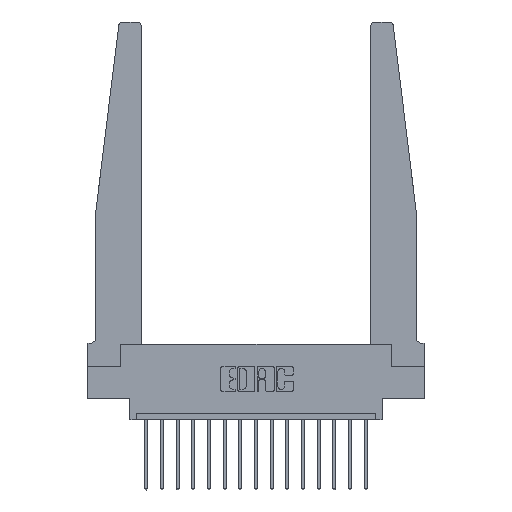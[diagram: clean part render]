
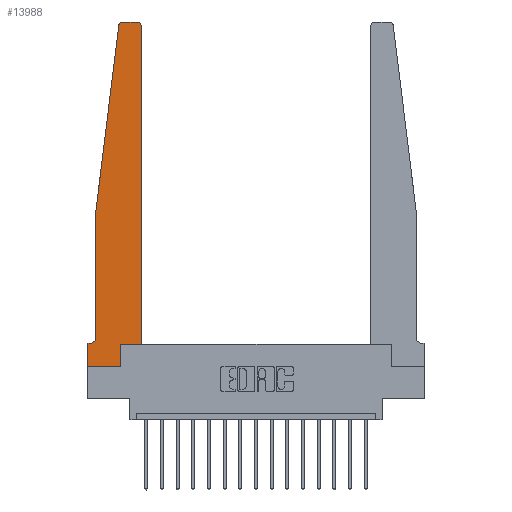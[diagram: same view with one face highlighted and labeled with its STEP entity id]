
A CAD part, top view. The second image highlights one B-rep face of the part: STEP entity #13988.
In plain terms, the highlighted planar face has unit normal (0, 0, 1).
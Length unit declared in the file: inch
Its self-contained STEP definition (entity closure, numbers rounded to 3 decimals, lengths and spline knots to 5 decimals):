
#480 = CARTESIAN_POINT ( 'NONE',  ( 0.065, 1.25, 0.37 ) ) ;
#621 = CARTESIAN_POINT ( 'NONE',  ( 0., 0.1875, 0.37 ) ) ;
#783 = CARTESIAN_POINT ( 'NONE',  ( 0.395, 2.75, 0.37 ) ) ;
#1248 = DIRECTION ( 'NONE',  ( 1., 0., 0. ) ) ;
#1488 = ORIENTED_EDGE ( 'NONE', *, *, #14935, .T. ) ;
#1908 = VERTEX_POINT ( 'NONE', #783 ) ;
#2038 = DIRECTION ( 'NONE',  ( -1., 0., 0. ) ) ;
#2104 = VERTEX_POINT ( 'NONE', #3308 ) ;
#2433 = ORIENTED_EDGE ( 'NONE', *, *, #8344, .T. ) ;
#2502 = LINE ( 'NONE', #14557, #13709 ) ;
#2522 = CIRCLE ( 'NONE', #10363, 0.05 ) ;
#2773 = VECTOR ( 'NONE', #1248, 39.37008 ) ;
#3038 = VERTEX_POINT ( 'NONE', #7591 ) ;
#3308 = CARTESIAN_POINT ( 'NONE',  ( 0., 0.1875, 0.37 ) ) ;
#3406 = CARTESIAN_POINT ( 'NONE',  ( 0.2605, 0.18, 0.37 ) ) ;
#3491 = VERTEX_POINT ( 'NONE', #6097 ) ;
#3689 = ORIENTED_EDGE ( 'NONE', *, *, #9313, .T. ) ;
#3926 = CARTESIAN_POINT ( 'NONE',  ( 0.065, 1.25, 0.37 ) ) ;
#4553 = VECTOR ( 'NONE', #16509, 39.37008 ) ;
#4703 = DIRECTION ( 'NONE',  ( 0., 1., 0. ) ) ;
#4928 = EDGE_CURVE ( 'NONE', #1908, #5959, #12519, .T. ) ;
#5096 = EDGE_CURVE ( 'NONE', #12871, #5785, #17444, .T. ) ;
#5451 = EDGE_CURVE ( 'NONE', #3491, #14314, #6489, .T. ) ;
#5543 = DIRECTION ( 'NONE',  ( 0., -1., 0. ) ) ;
#5785 = VERTEX_POINT ( 'NONE', #13978 ) ;
#5904 = ORIENTED_EDGE ( 'NONE', *, *, #12366, .T. ) ;
#5959 = VERTEX_POINT ( 'NONE', #14823 ) ;
#6097 = CARTESIAN_POINT ( 'NONE',  ( 0., 0., 0.37 ) ) ;
#6121 = DIRECTION ( 'NONE',  ( 0., 0., 1. ) ) ;
#6227 = DIRECTION ( 'NONE',  ( 0., 1., 0. ) ) ;
#6236 = CARTESIAN_POINT ( 'NONE',  ( 0.425, 2.72, 0.37 ) ) ;
#6269 = CARTESIAN_POINT ( 'NONE',  ( 0.015, 0.2375, 0.37 ) ) ;
#6274 = CARTESIAN_POINT ( 'NONE',  ( 0., 0., 0.37 ) ) ;
#6448 = DIRECTION ( 'NONE',  ( 1., 0., 0. ) ) ;
#6489 = LINE ( 'NONE', #6274, #15973 ) ;
#6546 = CARTESIAN_POINT ( 'NONE',  ( 0.24675, 2.72367, 0.37 ) ) ;
#6833 = CARTESIAN_POINT ( 'NONE',  ( 0.25, 2.75, 0.37 ) ) ;
#6857 = EDGE_CURVE ( 'NONE', #11253, #3038, #9467, .T. ) ;
#6870 = AXIS2_PLACEMENT_3D ( 'NONE', #11868, #9277, #6448 ) ;
#6974 = VERTEX_POINT ( 'NONE', #12579 ) ;
#6988 = AXIS2_PLACEMENT_3D ( 'NONE', #621, #6121, #8669 ) ;
#7047 = LINE ( 'NONE', #9644, #16525 ) ;
#7120 = DIRECTION ( 'NONE',  ( 1., 0., 0. ) ) ;
#7545 = CARTESIAN_POINT ( 'NONE',  ( 0.2605, 0.18, 0.37 ) ) ;
#7557 = EDGE_CURVE ( 'NONE', #2104, #3491, #7047, .T. ) ;
#7591 = CARTESIAN_POINT ( 'NONE',  ( 0.425, 0.18, 0.37 ) ) ;
#7655 = DIRECTION ( 'NONE',  ( 0., 0., -1. ) ) ;
#8344 = EDGE_CURVE ( 'NONE', #6974, #2104, #2502, .T. ) ;
#8518 = VECTOR ( 'NONE', #4703, 39.37008 ) ;
#8548 = ORIENTED_EDGE ( 'NONE', *, *, #16990, .T. ) ;
#8644 = LINE ( 'NONE', #7545, #16201 ) ;
#8669 = DIRECTION ( 'NONE',  ( 1., 0., 0. ) ) ;
#9277 = DIRECTION ( 'NONE',  ( 0., 0., 1. ) ) ;
#9313 = EDGE_CURVE ( 'NONE', #3038, #16264, #12194, .T. ) ;
#9467 = LINE ( 'NONE', #17684, #2773 ) ;
#9644 = CARTESIAN_POINT ( 'NONE',  ( 0., 0., 0.37 ) ) ;
#9719 = ORIENTED_EDGE ( 'NONE', *, *, #5451, .T. ) ;
#9935 = CARTESIAN_POINT ( 'NONE',  ( 0.2605, 0., 0.37 ) ) ;
#9998 = DIRECTION ( 'NONE',  ( 0., -1., 0. ) ) ;
#10363 = AXIS2_PLACEMENT_3D ( 'NONE', #6269, #7655, #17209 ) ;
#10529 = FACE_OUTER_BOUND ( 'NONE', #15155, .T. ) ;
#10700 = CIRCLE ( 'NONE', #16683, 0.03 ) ;
#10839 = LINE ( 'NONE', #17429, #15358 ) ;
#11007 = EDGE_CURVE ( 'NONE', #14314, #11253, #8644, .T. ) ;
#11041 = ORIENTED_EDGE ( 'NONE', *, *, #11007, .T. ) ;
#11253 = VERTEX_POINT ( 'NONE', #3406 ) ;
#11341 = DIRECTION ( 'NONE',  ( 0., 0., 1. ) ) ;
#11452 = ORIENTED_EDGE ( 'NONE', *, *, #5096, .T. ) ;
#11868 = CARTESIAN_POINT ( 'NONE',  ( 0.27653, 2.72, 0.37 ) ) ;
#12055 = CIRCLE ( 'NONE', #6870, 0.03 ) ;
#12194 = LINE ( 'NONE', #14048, #8518 ) ;
#12366 = EDGE_CURVE ( 'NONE', #5959, #14798, #12055, .T. ) ;
#12519 = LINE ( 'NONE', #6833, #4553 ) ;
#12579 = CARTESIAN_POINT ( 'NONE',  ( 0.015, 0.1875, 0.37 ) ) ;
#12871 = VERTEX_POINT ( 'NONE', #3926 ) ;
#13558 = EDGE_CURVE ( 'NONE', #5785, #6974, #2522, .T. ) ;
#13709 = VECTOR ( 'NONE', #2038, 39.37008 ) ;
#13826 = VECTOR ( 'NONE', #9998, 39.37008 ) ;
#13978 = CARTESIAN_POINT ( 'NONE',  ( 0.065, 0.2375, 0.37 ) ) ;
#13988 = ADVANCED_FACE ( 'NONE', ( #10529 ), #15545, .T. ) ;
#14048 = CARTESIAN_POINT ( 'NONE',  ( 0.425, 0.18, 0.37 ) ) ;
#14314 = VERTEX_POINT ( 'NONE', #9935 ) ;
#14557 = CARTESIAN_POINT ( 'NONE',  ( 0.065, 0.1875, 0.37 ) ) ;
#14798 = VERTEX_POINT ( 'NONE', #6546 ) ;
#14823 = CARTESIAN_POINT ( 'NONE',  ( 0.27653, 2.75, 0.37 ) ) ;
#14935 = EDGE_CURVE ( 'NONE', #16264, #1908, #10700, .T. ) ;
#15155 = EDGE_LOOP ( 'NONE', ( #15226, #5904, #8548, #11452, #17633, #2433, #17727, #9719, #11041, #15281, #3689, #1488 ) ) ;
#15226 = ORIENTED_EDGE ( 'NONE', *, *, #4928, .T. ) ;
#15281 = ORIENTED_EDGE ( 'NONE', *, *, #6857, .T. ) ;
#15358 = VECTOR ( 'NONE', #16026, 39.37008 ) ;
#15545 = PLANE ( 'NONE',  #6988 ) ;
#15973 = VECTOR ( 'NONE', #15980, 39.37008 ) ;
#15980 = DIRECTION ( 'NONE',  ( 1., 0., 0. ) ) ;
#16026 = DIRECTION ( 'NONE',  ( -0.122, -0.992, 0. ) ) ;
#16201 = VECTOR ( 'NONE', #6227, 39.37008 ) ;
#16264 = VERTEX_POINT ( 'NONE', #6236 ) ;
#16509 = DIRECTION ( 'NONE',  ( -1., 0., 0. ) ) ;
#16525 = VECTOR ( 'NONE', #5543, 39.37008 ) ;
#16683 = AXIS2_PLACEMENT_3D ( 'NONE', #16907, #11341, #7120 ) ;
#16907 = CARTESIAN_POINT ( 'NONE',  ( 0.395, 2.72, 0.37 ) ) ;
#16990 = EDGE_CURVE ( 'NONE', #14798, #12871, #10839, .T. ) ;
#17209 = DIRECTION ( 'NONE',  ( -1., 0., 0. ) ) ;
#17429 = CARTESIAN_POINT ( 'NONE',  ( 0.065, 1.25, 0.37 ) ) ;
#17444 = LINE ( 'NONE', #480, #13826 ) ;
#17633 = ORIENTED_EDGE ( 'NONE', *, *, #13558, .T. ) ;
#17684 = CARTESIAN_POINT ( 'NONE',  ( 0.425, 0.18, 0.37 ) ) ;
#17727 = ORIENTED_EDGE ( 'NONE', *, *, #7557, .T. ) ;
